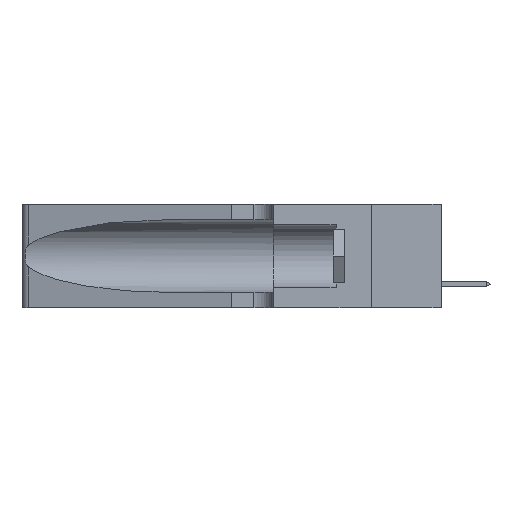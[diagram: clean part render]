
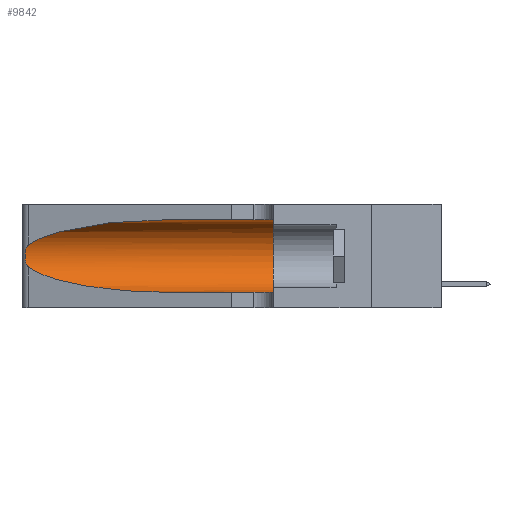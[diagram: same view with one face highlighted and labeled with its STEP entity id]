
A CAD part, left-side view. The second image highlights one B-rep face of the part: STEP entity #9842.
In plain terms, the highlighted cylindrical face has radius 3.308 mm (diameter 6.617 mm), a partial arc.
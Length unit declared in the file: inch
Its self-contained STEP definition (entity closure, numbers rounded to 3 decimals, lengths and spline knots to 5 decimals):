
#290 = VERTEX_POINT ( 'NONE', #20423 ) ;
#758 = CARTESIAN_POINT ( 'NONE',  ( 0.25487, 1.22718, 0.14631 ) ) ;
#912 = CARTESIAN_POINT ( 'NONE',  ( 0.1305, 0.35, 0.05475 ) ) ;
#1057 = DIRECTION ( 'NONE',  ( 0., -1., 0. ) ) ;
#1506 = FACE_OUTER_BOUND ( 'NONE', #19229, .T. ) ;
#1582 = CARTESIAN_POINT ( 'NONE',  ( 0.1305, 0.35, 0.185 ) ) ;
#1682 =( BOUNDED_CURVE ( )  B_SPLINE_CURVE ( 3, ( #25640, #23427, #2505, #27632 ),
 .UNSPECIFIED., .F., .F. ) 
 B_SPLINE_CURVE_WITH_KNOTS ( ( 4, 4 ),
 ( 1.5708, 2.84003 ),
 .UNSPECIFIED. ) 
 CURVE ( )  GEOMETRIC_REPRESENTATION_ITEM ( )  RATIONAL_B_SPLINE_CURVE ( ( 1., 0.87, 0.87, 1. ) ) 
 REPRESENTATION_ITEM ( '' )  );
#2115 = LINE ( 'NONE', #5801, #14258 ) ;
#2505 = CARTESIAN_POINT ( 'NONE',  ( 0.2373, 1.15595, 0.28018 ) ) ;
#2948 = ORIENTED_EDGE ( 'NONE', *, *, #26977, .F. ) ;
#3012 = CARTESIAN_POINT ( 'NONE',  ( 0.25487, 1.22718, 0.22369 ) ) ;
#3278 = CARTESIAN_POINT ( 'NONE',  ( 0.1305, 0.72297, 0.05475 ) ) ;
#3462 = EDGE_CURVE ( 'NONE', #4513, #26231, #10617, .T. ) ;
#3764 = DIRECTION ( 'NONE',  ( 0., 1., 0. ) ) ;
#4513 = VERTEX_POINT ( 'NONE', #28301 ) ;
#4766 =( BOUNDED_CURVE ( )  B_SPLINE_CURVE ( 3, ( #5347, #12243, #12429, #3278 ),
 .UNSPECIFIED., .F., .F. ) 
 B_SPLINE_CURVE_WITH_KNOTS ( ( 4, 4 ),
 ( 3.44316, 4.71239 ),
 .UNSPECIFIED. ) 
 CURVE ( )  GEOMETRIC_REPRESENTATION_ITEM ( )  RATIONAL_B_SPLINE_CURVE ( ( 1., 0.87, 0.87, 1. ) ) 
 REPRESENTATION_ITEM ( '' )  );
#5283 = CARTESIAN_POINT ( 'NONE',  ( 0.26075, 1.23896, 0.19203 ) ) ;
#5347 = CARTESIAN_POINT ( 'NONE',  ( 0.25487, 1.22718, 0.14631 ) ) ;
#5801 = CARTESIAN_POINT ( 'NONE',  ( 0.1305, 1.61858, 0.05475 ) ) ;
#7296 = CIRCLE ( 'NONE', #19793, 0.13025 ) ;
#7599 = CARTESIAN_POINT ( 'NONE',  ( 0.25487, 1.22718, 0.14631 ) ) ;
#7607 = CARTESIAN_POINT ( 'NONE',  ( 0.1305, 1.61858, 0.185 ) ) ;
#7867 = VECTOR ( 'NONE', #27413, 39.37008 ) ;
#8597 = EDGE_CURVE ( 'NONE', #26231, #12019, #4766, .T. ) ;
#8825 = CARTESIAN_POINT ( 'NONE',  ( 0.1305, 0.72297, 0.05475 ) ) ;
#9842 = ADVANCED_FACE ( 'NONE', ( #1506 ), #19675, .F. ) ;
#9890 = CARTESIAN_POINT ( 'NONE',  ( 0.26018, 1.23835, 0.19895 ) ) ;
#10617 = B_SPLINE_CURVE_WITH_KNOTS ( 'NONE', 3,
 ( #3012, #28145, #21519, #16959, #12276, #9890, #5283, #14474, #18962, #23833, #21224, #14670, #16649, #7599 ),
 .UNSPECIFIED., .F., .F.,
 ( 4, 2, 2, 2, 2, 2, 4 ),
 ( 0., 0.00027, 0.00053, 0.00107, 0.0016, 0.00187, 0.00214 ),
 .UNSPECIFIED. ) ;
#11361 = CARTESIAN_POINT ( 'NONE',  ( 0.1305, 1.61858, 0.31525 ) ) ;
#12019 = VERTEX_POINT ( 'NONE', #8825 ) ;
#12074 = DIRECTION ( 'NONE',  ( 0., -1., 0. ) ) ;
#12161 = ORIENTED_EDGE ( 'NONE', *, *, #23853, .F. ) ;
#12243 = CARTESIAN_POINT ( 'NONE',  ( 0.2373, 1.15595, 0.08982 ) ) ;
#12276 = CARTESIAN_POINT ( 'NONE',  ( 0.25854, 1.2359, 0.20912 ) ) ;
#12429 = CARTESIAN_POINT ( 'NONE',  ( 0.18966, 0.96281, 0.05475 ) ) ;
#12973 = ORIENTED_EDGE ( 'NONE', *, *, #8597, .T. ) ;
#14258 = VECTOR ( 'NONE', #1057, 39.37008 ) ;
#14474 = CARTESIAN_POINT ( 'NONE',  ( 0.26075, 1.23896, 0.178 ) ) ;
#14670 = CARTESIAN_POINT ( 'NONE',  ( 0.25639, 1.23186, 0.15144 ) ) ;
#15602 = ORIENTED_EDGE ( 'NONE', *, *, #17945, .T. ) ;
#16649 = CARTESIAN_POINT ( 'NONE',  ( 0.25555, 1.22993, 0.14849 ) ) ;
#16959 = CARTESIAN_POINT ( 'NONE',  ( 0.25787, 1.23484, 0.2124 ) ) ;
#17417 = ORIENTED_EDGE ( 'NONE', *, *, #3462, .T. ) ;
#17532 = EDGE_CURVE ( 'NONE', #12019, #24053, #2115, .T. ) ;
#17945 = EDGE_CURVE ( 'NONE', #23757, #4513, #1682, .T. ) ;
#18205 = ORIENTED_EDGE ( 'NONE', *, *, #17532, .T. ) ;
#18962 = CARTESIAN_POINT ( 'NONE',  ( 0.26017, 1.23833, 0.17102 ) ) ;
#19229 = EDGE_LOOP ( 'NONE', ( #15602, #17417, #12973, #18205, #2948, #12161 ) ) ;
#19675 = CYLINDRICAL_SURFACE ( 'NONE', #26978, 0.13025 ) ;
#19702 = DIRECTION ( 'NONE',  ( 0., 0., 1. ) ) ;
#19793 = AXIS2_PLACEMENT_3D ( 'NONE', #1582, #3764, #19702 ) ;
#20423 = CARTESIAN_POINT ( 'NONE',  ( 0.1305, 0.35, 0.31525 ) ) ;
#21224 = CARTESIAN_POINT ( 'NONE',  ( 0.25789, 1.23486, 0.15765 ) ) ;
#21519 = CARTESIAN_POINT ( 'NONE',  ( 0.25639, 1.23184, 0.21858 ) ) ;
#23427 = CARTESIAN_POINT ( 'NONE',  ( 0.18966, 0.96281, 0.31525 ) ) ;
#23540 = DIRECTION ( 'NONE',  ( 0., 0., -1. ) ) ;
#23757 = VERTEX_POINT ( 'NONE', #29236 ) ;
#23833 = CARTESIAN_POINT ( 'NONE',  ( 0.25856, 1.23593, 0.16098 ) ) ;
#23853 = EDGE_CURVE ( 'NONE', #23757, #290, #27111, .T. ) ;
#24053 = VERTEX_POINT ( 'NONE', #912 ) ;
#25640 = CARTESIAN_POINT ( 'NONE',  ( 0.1305, 0.72297, 0.31525 ) ) ;
#26231 = VERTEX_POINT ( 'NONE', #758 ) ;
#26977 = EDGE_CURVE ( 'NONE', #290, #24053, #7296, .T. ) ;
#26978 = AXIS2_PLACEMENT_3D ( 'NONE', #7607, #12074, #23540 ) ;
#27111 = LINE ( 'NONE', #11361, #7867 ) ;
#27413 = DIRECTION ( 'NONE',  ( 0., -1., 0. ) ) ;
#27632 = CARTESIAN_POINT ( 'NONE',  ( 0.25487, 1.22718, 0.22369 ) ) ;
#28145 = CARTESIAN_POINT ( 'NONE',  ( 0.25555, 1.22994, 0.2215 ) ) ;
#28301 = CARTESIAN_POINT ( 'NONE',  ( 0.25487, 1.22718, 0.22369 ) ) ;
#29236 = CARTESIAN_POINT ( 'NONE',  ( 0.1305, 0.72297, 0.31525 ) ) ;
